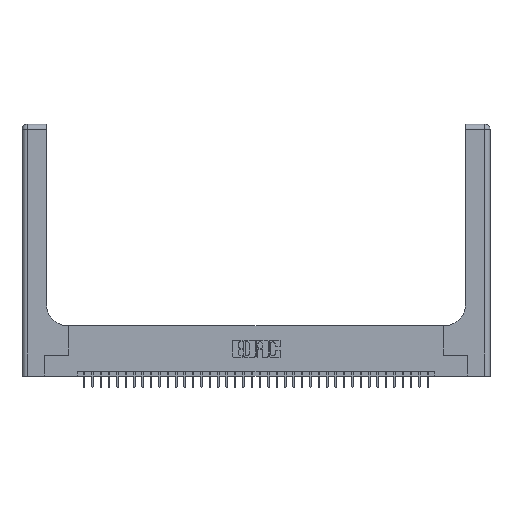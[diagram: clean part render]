
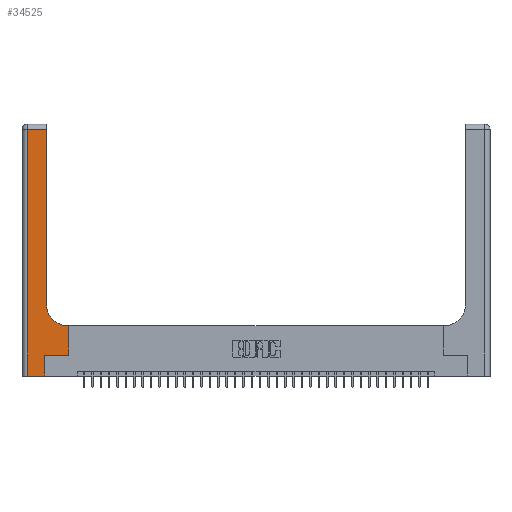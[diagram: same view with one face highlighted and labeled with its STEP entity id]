
A CAD part, top view. The second image highlights one B-rep face of the part: STEP entity #34525.
In plain terms, the highlighted planar face has unit normal (0, 0, 1).
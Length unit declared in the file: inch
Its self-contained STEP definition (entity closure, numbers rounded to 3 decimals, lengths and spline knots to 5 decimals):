
#524 = DIRECTION ( 'NONE',  ( 0., 1., 0. ) ) ;
#1099 = ORIENTED_EDGE ( 'NONE', *, *, #16052, .T. ) ;
#2149 = VECTOR ( 'NONE', #26847, 39.37008 ) ;
#2274 = CARTESIAN_POINT ( 'NONE',  ( 0.5585, 0.6, 0.37 ) ) ;
#2659 = VERTEX_POINT ( 'NONE', #30404 ) ;
#3123 = LINE ( 'NONE', #20010, #34764 ) ;
#3224 = CARTESIAN_POINT ( 'NONE',  ( 0.2915, 0.6, 0.37 ) ) ;
#3836 = VECTOR ( 'NONE', #17224, 39.37008 ) ;
#4014 = EDGE_LOOP ( 'NONE', ( #25928, #13223, #26807, #33552, #1099, #12189, #14581, #16573, #36366 ) ) ;
#4587 = VECTOR ( 'NONE', #10863, 39.37008 ) ;
#4610 = DIRECTION ( 'NONE',  ( 0., 1., 0. ) ) ;
#4897 = DIRECTION ( 'NONE',  ( 0., 0., -1. ) ) ;
#4975 = PLANE ( 'NONE',  #12729 ) ;
#5315 = VERTEX_POINT ( 'NONE', #5638 ) ;
#5638 = CARTESIAN_POINT ( 'NONE',  ( 0.5585, 0.25, 0.37 ) ) ;
#6978 = VERTEX_POINT ( 'NONE', #7550 ) ;
#7509 = LINE ( 'NONE', #19302, #31151 ) ;
#7550 = CARTESIAN_POINT ( 'NONE',  ( 0.269, 0.25, 0.37 ) ) ;
#8771 = VECTOR ( 'NONE', #524, 39.37008 ) ;
#8846 = DIRECTION ( 'NONE',  ( 0., 1., 0. ) ) ;
#9049 = CARTESIAN_POINT ( 'NONE',  ( 0.2915, 3., 0.37 ) ) ;
#9904 = EDGE_CURVE ( 'NONE', #6978, #5315, #3123, .T. ) ;
#10114 = EDGE_CURVE ( 'NONE', #33993, #2659, #27885, .T. ) ;
#10265 = CIRCLE ( 'NONE', #37452, 0.25 ) ;
#10863 = DIRECTION ( 'NONE',  ( 0., -1., 0. ) ) ;
#11175 = CARTESIAN_POINT ( 'NONE',  ( 0.06, 0., 0.37 ) ) ;
#11569 = LINE ( 'NONE', #9049, #29467 ) ;
#12080 = CARTESIAN_POINT ( 'NONE',  ( 0.2915, 0.85, 0.37 ) ) ;
#12189 = ORIENTED_EDGE ( 'NONE', *, *, #9904, .T. ) ;
#12410 = VERTEX_POINT ( 'NONE', #34744 ) ;
#12729 = AXIS2_PLACEMENT_3D ( 'NONE', #28594, #31688, #28803 ) ;
#13223 = ORIENTED_EDGE ( 'NONE', *, *, #10114, .T. ) ;
#13814 = VERTEX_POINT ( 'NONE', #12080 ) ;
#14178 = LINE ( 'NONE', #31039, #21184 ) ;
#14581 = ORIENTED_EDGE ( 'NONE', *, *, #31851, .T. ) ;
#14628 = VERTEX_POINT ( 'NONE', #11175 ) ;
#14726 = EDGE_CURVE ( 'NONE', #34549, #17192, #29758, .T. ) ;
#15111 = DIRECTION ( 'NONE',  ( 1., 0., 0. ) ) ;
#16052 = EDGE_CURVE ( 'NONE', #12410, #6978, #18686, .T. ) ;
#16513 = DIRECTION ( 'NONE',  ( 1., 0., 0. ) ) ;
#16573 = ORIENTED_EDGE ( 'NONE', *, *, #14726, .T. ) ;
#17192 = VERTEX_POINT ( 'NONE', #29236 ) ;
#17224 = DIRECTION ( 'NONE',  ( -1., 0., 0. ) ) ;
#18686 = LINE ( 'NONE', #27236, #8771 ) ;
#19302 = CARTESIAN_POINT ( 'NONE',  ( 0.5585, 0.25, 0.37 ) ) ;
#20010 = CARTESIAN_POINT ( 'NONE',  ( 0.269, 0.25, 0.37 ) ) ;
#20068 = FACE_OUTER_BOUND ( 'NONE', #4014, .T. ) ;
#21184 = VECTOR ( 'NONE', #16513, 39.37008 ) ;
#22430 = CARTESIAN_POINT ( 'NONE',  ( 0.2915, 2.94, 0.37 ) ) ;
#25071 = EDGE_CURVE ( 'NONE', #13814, #33993, #11569, .T. ) ;
#25126 = EDGE_CURVE ( 'NONE', #17192, #13814, #10265, .T. ) ;
#25580 = LINE ( 'NONE', #37383, #4587 ) ;
#25928 = ORIENTED_EDGE ( 'NONE', *, *, #25071, .T. ) ;
#26807 = ORIENTED_EDGE ( 'NONE', *, *, #28619, .T. ) ;
#26847 = DIRECTION ( 'NONE',  ( -1., 0., 0. ) ) ;
#27065 = EDGE_CURVE ( 'NONE', #14628, #12410, #14178, .T. ) ;
#27236 = CARTESIAN_POINT ( 'NONE',  ( 0.269, 0., 0.37 ) ) ;
#27885 = LINE ( 'NONE', #36785, #3836 ) ;
#28594 = CARTESIAN_POINT ( 'NONE',  ( 0., 3., 0.37 ) ) ;
#28619 = EDGE_CURVE ( 'NONE', #2659, #14628, #25580, .T. ) ;
#28803 = DIRECTION ( 'NONE',  ( -1., 0., 0. ) ) ;
#29236 = CARTESIAN_POINT ( 'NONE',  ( 0.5415, 0.6, 0.37 ) ) ;
#29467 = VECTOR ( 'NONE', #8846, 39.37008 ) ;
#29758 = LINE ( 'NONE', #3224, #2149 ) ;
#30404 = CARTESIAN_POINT ( 'NONE',  ( 0.06, 2.94, 0.37 ) ) ;
#31039 = CARTESIAN_POINT ( 'NONE',  ( 0., 0., 0.37 ) ) ;
#31151 = VECTOR ( 'NONE', #4610, 39.37008 ) ;
#31688 = DIRECTION ( 'NONE',  ( 0., 0., -1. ) ) ;
#31851 = EDGE_CURVE ( 'NONE', #5315, #34549, #7509, .T. ) ;
#33552 = ORIENTED_EDGE ( 'NONE', *, *, #27065, .T. ) ;
#33993 = VERTEX_POINT ( 'NONE', #22430 ) ;
#34326 = DIRECTION ( 'NONE',  ( 1., 0., 0. ) ) ;
#34525 = ADVANCED_FACE ( 'NONE', ( #20068 ), #4975, .F. ) ;
#34549 = VERTEX_POINT ( 'NONE', #2274 ) ;
#34744 = CARTESIAN_POINT ( 'NONE',  ( 0.269, 0., 0.37 ) ) ;
#34764 = VECTOR ( 'NONE', #15111, 39.37008 ) ;
#36315 = CARTESIAN_POINT ( 'NONE',  ( 0.5415, 0.85, 0.37 ) ) ;
#36366 = ORIENTED_EDGE ( 'NONE', *, *, #25126, .T. ) ;
#36785 = CARTESIAN_POINT ( 'NONE',  ( 0., 2.94, 0.37 ) ) ;
#37383 = CARTESIAN_POINT ( 'NONE',  ( 0.06, 3., 0.37 ) ) ;
#37452 = AXIS2_PLACEMENT_3D ( 'NONE', #36315, #4897, #34326 ) ;
